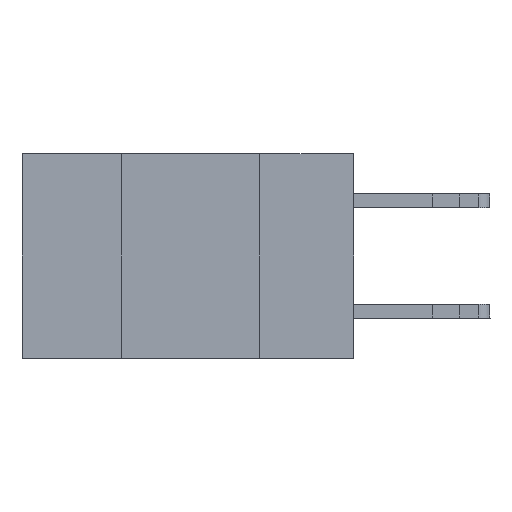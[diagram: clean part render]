
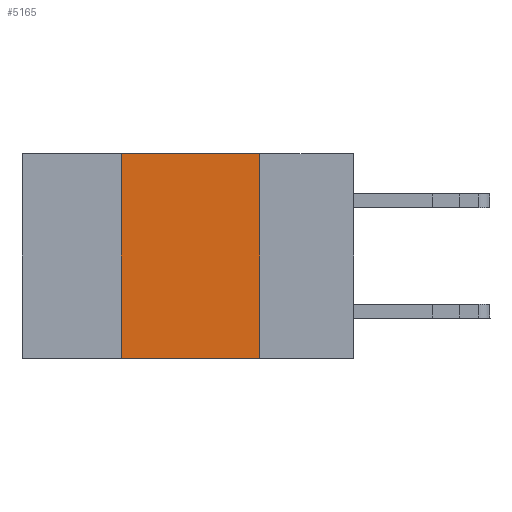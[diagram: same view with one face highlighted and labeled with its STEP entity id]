
A CAD part, left-side view. The second image highlights one B-rep face of the part: STEP entity #5165.
In plain terms, the highlighted planar face has unit normal (-1, 0, 0).
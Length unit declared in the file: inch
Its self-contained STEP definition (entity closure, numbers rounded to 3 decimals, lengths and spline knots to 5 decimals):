
#178 = LINE ( 'NONE', #3171, #15720 ) ;
#590 = FACE_OUTER_BOUND ( 'NONE', #8352, .T. ) ;
#1800 = VECTOR ( 'NONE', #18144, 39.37008 ) ;
#2369 = CARTESIAN_POINT ( 'NONE',  ( 0., 0.6, 0. ) ) ;
#2583 = CARTESIAN_POINT ( 'NONE',  ( 0., 0.6, 0. ) ) ;
#3171 = CARTESIAN_POINT ( 'NONE',  ( 0., 0.17, 0. ) ) ;
#3229 = EDGE_CURVE ( 'NONE', #15471, #12147, #14558, .T. ) ;
#4088 = DIRECTION ( 'NONE',  ( 1., 0., 0. ) ) ;
#4737 = CARTESIAN_POINT ( 'NONE',  ( 0., 0.17, 0. ) ) ;
#5024 = ORIENTED_EDGE ( 'NONE', *, *, #3229, .F. ) ;
#5165 = ADVANCED_FACE ( 'NONE', ( #590 ), #11632, .F. ) ;
#5797 = LINE ( 'NONE', #9266, #1800 ) ;
#6019 = EDGE_CURVE ( 'NONE', #15471, #11638, #5797, .T. ) ;
#6724 = LINE ( 'NONE', #2369, #10262 ) ;
#8352 = EDGE_LOOP ( 'NONE', ( #12803, #16320, #5024, #11860 ) ) ;
#9266 = CARTESIAN_POINT ( 'NONE',  ( 0., 0.6, -0.37 ) ) ;
#9445 = AXIS2_PLACEMENT_3D ( 'NONE', #2583, #4088, #14603 ) ;
#9901 = DIRECTION ( 'NONE',  ( 0., -1., 0. ) ) ;
#10262 = VECTOR ( 'NONE', #9901, 39.37008 ) ;
#10333 = CARTESIAN_POINT ( 'NONE',  ( 0., 0.17, -0.37 ) ) ;
#10596 = EDGE_CURVE ( 'NONE', #14774, #11638, #178, .T. ) ;
#11175 = DIRECTION ( 'NONE',  ( 0., 0., 1. ) ) ;
#11196 = CARTESIAN_POINT ( 'NONE',  ( 0., 0.42, 0. ) ) ;
#11442 = CARTESIAN_POINT ( 'NONE',  ( 0., 0.42, 0. ) ) ;
#11632 = PLANE ( 'NONE',  #9445 ) ;
#11638 = VERTEX_POINT ( 'NONE', #10333 ) ;
#11860 = ORIENTED_EDGE ( 'NONE', *, *, #6019, .T. ) ;
#12147 = VERTEX_POINT ( 'NONE', #11442 ) ;
#12314 = CARTESIAN_POINT ( 'NONE',  ( 0., 0.42, -0.37 ) ) ;
#12772 = EDGE_CURVE ( 'NONE', #12147, #14774, #6724, .T. ) ;
#12803 = ORIENTED_EDGE ( 'NONE', *, *, #10596, .F. ) ;
#14558 = LINE ( 'NONE', #11196, #18481 ) ;
#14603 = DIRECTION ( 'NONE',  ( 0., 0., -1. ) ) ;
#14774 = VERTEX_POINT ( 'NONE', #4737 ) ;
#15200 = DIRECTION ( 'NONE',  ( 0., 0., -1. ) ) ;
#15471 = VERTEX_POINT ( 'NONE', #12314 ) ;
#15720 = VECTOR ( 'NONE', #15200, 39.37008 ) ;
#16320 = ORIENTED_EDGE ( 'NONE', *, *, #12772, .F. ) ;
#18144 = DIRECTION ( 'NONE',  ( 0., -1., 0. ) ) ;
#18481 = VECTOR ( 'NONE', #11175, 39.37008 ) ;
